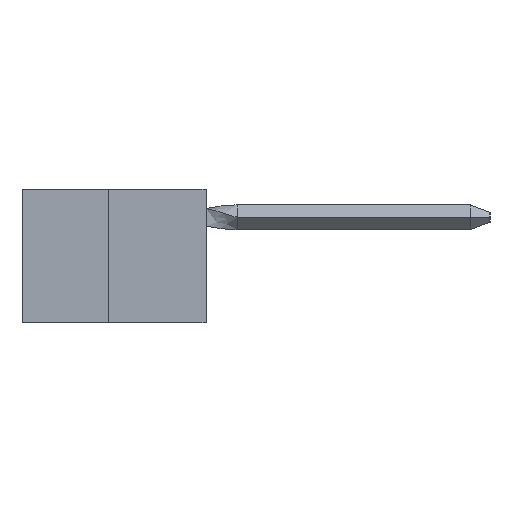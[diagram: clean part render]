
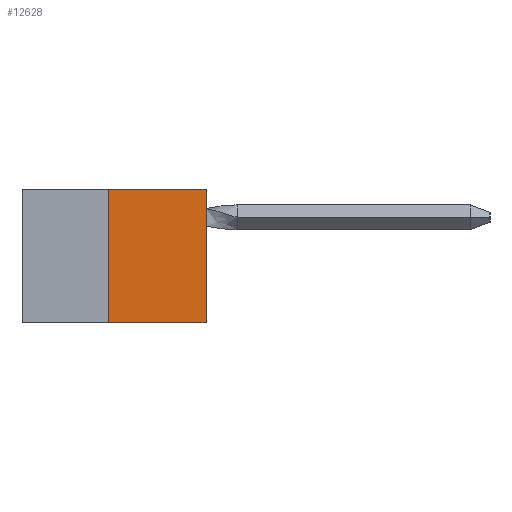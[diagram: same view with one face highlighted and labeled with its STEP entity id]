
A CAD part, left-side view. The second image highlights one B-rep face of the part: STEP entity #12628.
In plain terms, the highlighted planar face has unit normal (-1, 0, 0).
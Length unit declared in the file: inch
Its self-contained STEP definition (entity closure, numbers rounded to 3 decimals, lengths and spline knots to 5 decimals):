
#1834 = EDGE_CURVE ( 'NONE', #18632, #5304, #28553, .T. ) ;
#2757 = LINE ( 'NONE', #27868, #3188 ) ;
#3188 = VECTOR ( 'NONE', #34391, 39.37008 ) ;
#5304 = VERTEX_POINT ( 'NONE', #27811 ) ;
#6188 = CARTESIAN_POINT ( 'NONE',  ( 0., 0., -0.343 ) ) ;
#7144 = VERTEX_POINT ( 'NONE', #6188 ) ;
#7561 = VECTOR ( 'NONE', #34401, 39.37008 ) ;
#8094 = LINE ( 'NONE', #28764, #7561 ) ;
#8120 = LINE ( 'NONE', #9130, #22915 ) ;
#8849 = DIRECTION ( 'NONE',  ( 0., 0., 1. ) ) ;
#9130 = CARTESIAN_POINT ( 'NONE',  ( 0., 0.473, -0.343 ) ) ;
#11786 = PLANE ( 'NONE',  #36730 ) ;
#12091 = DIRECTION ( 'NONE',  ( 0., -1., 0. ) ) ;
#12628 = ADVANCED_FACE ( 'NONE', ( #17569 ), #11786, .F. ) ;
#14577 = EDGE_CURVE ( 'NONE', #5304, #30417, #8094, .T. ) ;
#15258 = ORIENTED_EDGE ( 'NONE', *, *, #25834, .T. ) ;
#17569 = FACE_OUTER_BOUND ( 'NONE', #21951, .T. ) ;
#18632 = VERTEX_POINT ( 'NONE', #29806 ) ;
#21951 = EDGE_LOOP ( 'NONE', ( #28479, #26838, #15258, #24292 ) ) ;
#22915 = VECTOR ( 'NONE', #12091, 39.37008 ) ;
#24292 = ORIENTED_EDGE ( 'NONE', *, *, #30049, .T. ) ;
#25834 = EDGE_CURVE ( 'NONE', #18632, #7144, #8120, .T. ) ;
#26788 = CARTESIAN_POINT ( 'NONE',  ( 0., 0., 0. ) ) ;
#26838 = ORIENTED_EDGE ( 'NONE', *, *, #1834, .F. ) ;
#27811 = CARTESIAN_POINT ( 'NONE',  ( 0., 0.25, 0. ) ) ;
#27868 = CARTESIAN_POINT ( 'NONE',  ( 0., 0., 0. ) ) ;
#28479 = ORIENTED_EDGE ( 'NONE', *, *, #14577, .F. ) ;
#28553 = LINE ( 'NONE', #37107, #35434 ) ;
#28764 = CARTESIAN_POINT ( 'NONE',  ( 0., 0.473, 0. ) ) ;
#29705 = CARTESIAN_POINT ( 'NONE',  ( 0., 0.473, 0. ) ) ;
#29806 = CARTESIAN_POINT ( 'NONE',  ( 0., 0.25, -0.343 ) ) ;
#30049 = EDGE_CURVE ( 'NONE', #7144, #30417, #2757, .T. ) ;
#30417 = VERTEX_POINT ( 'NONE', #26788 ) ;
#32658 = DIRECTION ( 'NONE',  ( 0., 0., -1. ) ) ;
#34391 = DIRECTION ( 'NONE',  ( 0., 0., 1. ) ) ;
#34401 = DIRECTION ( 'NONE',  ( 0., -1., 0. ) ) ;
#35434 = VECTOR ( 'NONE', #8849, 39.37008 ) ;
#36730 = AXIS2_PLACEMENT_3D ( 'NONE', #29705, #38203, #32658 ) ;
#37107 = CARTESIAN_POINT ( 'NONE',  ( 0., 0.25, 0. ) ) ;
#38203 = DIRECTION ( 'NONE',  ( 1., 0., 0. ) ) ;
